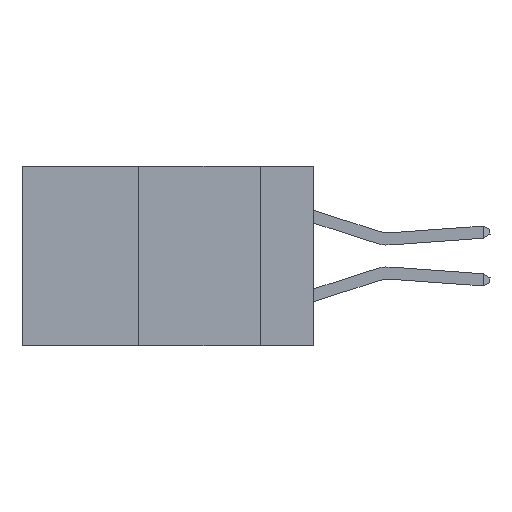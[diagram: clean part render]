
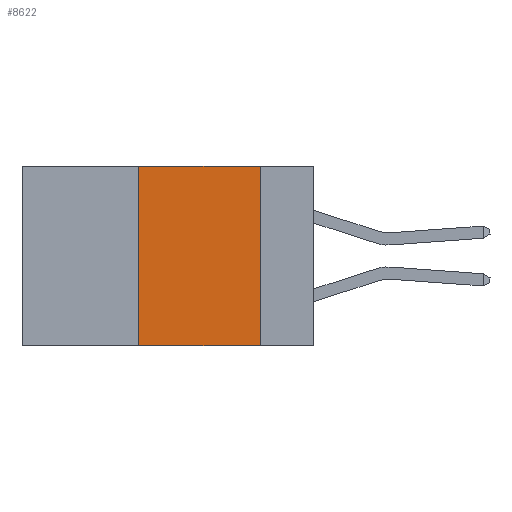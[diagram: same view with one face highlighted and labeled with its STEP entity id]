
A CAD part, left-side view. The second image highlights one B-rep face of the part: STEP entity #8622.
In plain terms, the highlighted planar face has unit normal (-1, 0, 0).
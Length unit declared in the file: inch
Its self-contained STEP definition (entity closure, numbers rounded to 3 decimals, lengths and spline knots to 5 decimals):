
#188 = AXIS2_PLACEMENT_3D ( 'NONE', #8582, #19096, #10129 ) ;
#207 = CARTESIAN_POINT ( 'NONE',  ( 0., 0.36, 0. ) ) ;
#412 = LINE ( 'NONE', #5655, #8474 ) ;
#1070 = DIRECTION ( 'NONE',  ( 0., -1., 0. ) ) ;
#2380 = LINE ( 'NONE', #10499, #10477 ) ;
#2477 = PLANE ( 'NONE',  #188 ) ;
#2705 = ORIENTED_EDGE ( 'NONE', *, *, #5804, .F. ) ;
#2910 = DIRECTION ( 'NONE',  ( 0., 0., -1. ) ) ;
#3543 = ORIENTED_EDGE ( 'NONE', *, *, #10465, .F. ) ;
#4184 = DIRECTION ( 'NONE',  ( 0., -1., 0. ) ) ;
#4224 = VECTOR ( 'NONE', #16955, 39.37008 ) ;
#4956 = LINE ( 'NONE', #19215, #8486 ) ;
#5655 = CARTESIAN_POINT ( 'NONE',  ( 0., 0.6, -0.37 ) ) ;
#5785 = EDGE_LOOP ( 'NONE', ( #2705, #3543, #13860, #7210 ) ) ;
#5804 = EDGE_CURVE ( 'NONE', #11225, #18750, #2380, .T. ) ;
#6859 = FACE_OUTER_BOUND ( 'NONE', #5785, .T. ) ;
#7210 = ORIENTED_EDGE ( 'NONE', *, *, #9186, .T. ) ;
#7269 = CARTESIAN_POINT ( 'NONE',  ( 0., 0.36, 0. ) ) ;
#8230 = LINE ( 'NONE', #207, #4224 ) ;
#8474 = VECTOR ( 'NONE', #1070, 39.37008 ) ;
#8486 = VECTOR ( 'NONE', #4184, 39.37008 ) ;
#8582 = CARTESIAN_POINT ( 'NONE',  ( 0., 0.6, 0. ) ) ;
#8622 = ADVANCED_FACE ( 'NONE', ( #6859 ), #2477, .F. ) ;
#8965 = EDGE_CURVE ( 'NONE', #9306, #18953, #8230, .T. ) ;
#9186 = EDGE_CURVE ( 'NONE', #9306, #18750, #412, .T. ) ;
#9306 = VERTEX_POINT ( 'NONE', #16472 ) ;
#10129 = DIRECTION ( 'NONE',  ( 0., 0., -1. ) ) ;
#10465 = EDGE_CURVE ( 'NONE', #18953, #11225, #4956, .T. ) ;
#10477 = VECTOR ( 'NONE', #2910, 39.37008 ) ;
#10499 = CARTESIAN_POINT ( 'NONE',  ( 0., 0.11, 0. ) ) ;
#11225 = VERTEX_POINT ( 'NONE', #14331 ) ;
#13860 = ORIENTED_EDGE ( 'NONE', *, *, #8965, .F. ) ;
#14331 = CARTESIAN_POINT ( 'NONE',  ( 0., 0.11, 0. ) ) ;
#14443 = CARTESIAN_POINT ( 'NONE',  ( 0., 0.11, -0.37 ) ) ;
#16472 = CARTESIAN_POINT ( 'NONE',  ( 0., 0.36, -0.37 ) ) ;
#16955 = DIRECTION ( 'NONE',  ( 0., 0., 1. ) ) ;
#18750 = VERTEX_POINT ( 'NONE', #14443 ) ;
#18953 = VERTEX_POINT ( 'NONE', #7269 ) ;
#19096 = DIRECTION ( 'NONE',  ( 1., 0., 0. ) ) ;
#19215 = CARTESIAN_POINT ( 'NONE',  ( 0., 0.6, 0. ) ) ;
